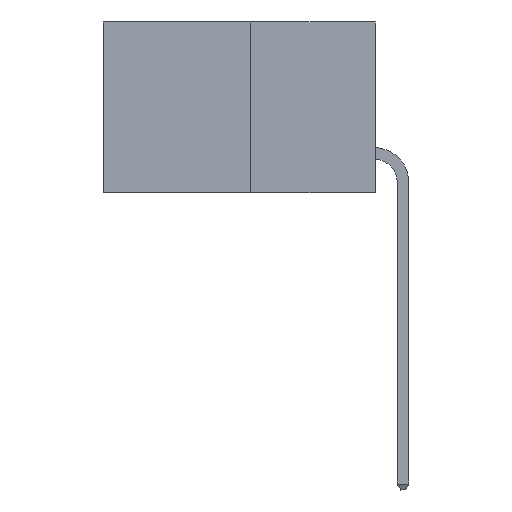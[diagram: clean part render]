
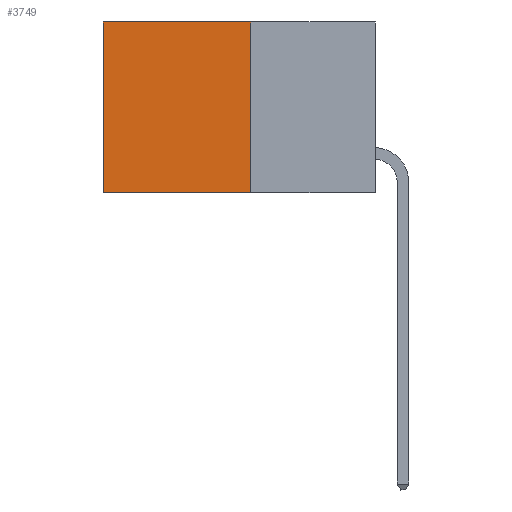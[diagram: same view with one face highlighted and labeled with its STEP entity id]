
A CAD part, left-side view. The second image highlights one B-rep face of the part: STEP entity #3749.
In plain terms, the highlighted planar face has unit normal (-1, 0, 0).
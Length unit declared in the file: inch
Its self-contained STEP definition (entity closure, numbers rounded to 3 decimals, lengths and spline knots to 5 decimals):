
#26 = VECTOR ( 'NONE', #9201, 39.37008 ) ;
#187 = EDGE_LOOP ( 'NONE', ( #6826, #6882, #7650, #7849 ) ) ;
#975 = VECTOR ( 'NONE', #8195, 39.37008 ) ;
#1382 = VERTEX_POINT ( 'NONE', #8871 ) ;
#1584 = FACE_OUTER_BOUND ( 'NONE', #187, .T. ) ;
#1728 = DIRECTION ( 'NONE',  ( 0., 0., -1. ) ) ;
#1760 = EDGE_CURVE ( 'NONE', #8592, #1382, #1885, .T. ) ;
#1885 = LINE ( 'NONE', #5985, #7188 ) ;
#3256 = LINE ( 'NONE', #7443, #5731 ) ;
#3749 = ADVANCED_FACE ( 'NONE', ( #1584 ), #5955, .F. ) ;
#5587 = CARTESIAN_POINT ( 'NONE',  ( 0.277, 0.27, -0.37 ) ) ;
#5731 = VECTOR ( 'NONE', #6394, 39.37008 ) ;
#5955 = PLANE ( 'NONE',  #10901 ) ;
#5985 = CARTESIAN_POINT ( 'NONE',  ( 0.277, 0.27, -0.37 ) ) ;
#6281 = DIRECTION ( 'NONE',  ( 0., 1., 0. ) ) ;
#6394 = DIRECTION ( 'NONE',  ( 0., 0., -1. ) ) ;
#6637 = CARTESIAN_POINT ( 'NONE',  ( 0.277, 0.59, 0. ) ) ;
#6675 = LINE ( 'NONE', #11200, #975 ) ;
#6826 = ORIENTED_EDGE ( 'NONE', *, *, #8916, .T. ) ;
#6882 = ORIENTED_EDGE ( 'NONE', *, *, #1760, .F. ) ;
#7188 = VECTOR ( 'NONE', #6281, 39.37008 ) ;
#7443 = CARTESIAN_POINT ( 'NONE',  ( 0.277, 0.27, -0.37 ) ) ;
#7650 = ORIENTED_EDGE ( 'NONE', *, *, #9735, .F. ) ;
#7849 = ORIENTED_EDGE ( 'NONE', *, *, #9534, .T. ) ;
#8077 = DIRECTION ( 'NONE',  ( 1., 0., 0. ) ) ;
#8195 = DIRECTION ( 'NONE',  ( 0., 1., 0. ) ) ;
#8592 = VERTEX_POINT ( 'NONE', #5587 ) ;
#8616 = VERTEX_POINT ( 'NONE', #6637 ) ;
#8661 = LINE ( 'NONE', #11173, #26 ) ;
#8871 = CARTESIAN_POINT ( 'NONE',  ( 0.277, 0.59, -0.37 ) ) ;
#8916 = EDGE_CURVE ( 'NONE', #8616, #1382, #8661, .T. ) ;
#9201 = DIRECTION ( 'NONE',  ( 0., 0., -1. ) ) ;
#9534 = EDGE_CURVE ( 'NONE', #11127, #8616, #6675, .T. ) ;
#9540 = CARTESIAN_POINT ( 'NONE',  ( 0.277, 0.27, 0. ) ) ;
#9735 = EDGE_CURVE ( 'NONE', #11127, #8592, #3256, .T. ) ;
#10901 = AXIS2_PLACEMENT_3D ( 'NONE', #12102, #8077, #1728 ) ;
#11127 = VERTEX_POINT ( 'NONE', #9540 ) ;
#11173 = CARTESIAN_POINT ( 'NONE',  ( 0.277, 0.59, -0.37 ) ) ;
#11200 = CARTESIAN_POINT ( 'NONE',  ( 0.277, 0.27, 0. ) ) ;
#12102 = CARTESIAN_POINT ( 'NONE',  ( 0.277, 0.27, -0.37 ) ) ;
